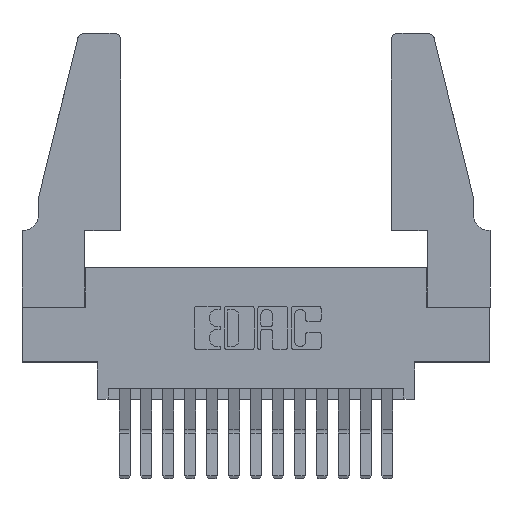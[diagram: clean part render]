
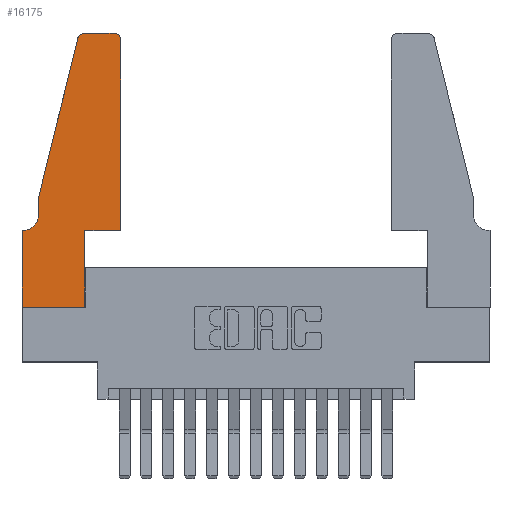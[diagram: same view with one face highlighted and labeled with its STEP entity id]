
A CAD part, top view. The second image highlights one B-rep face of the part: STEP entity #16175.
In plain terms, the highlighted planar face has unit normal (0, 0, 1).
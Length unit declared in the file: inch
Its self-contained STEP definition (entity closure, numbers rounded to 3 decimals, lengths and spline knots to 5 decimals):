
#160 = LINE ( 'NONE', #10211, #7240 ) ;
#206 = VERTEX_POINT ( 'NONE', #323 ) ;
#312 = CARTESIAN_POINT ( 'NONE',  ( 0.4205, 1.25, 0.37 ) ) ;
#323 = CARTESIAN_POINT ( 'NONE',  ( 0.2865, 0., 0.37 ) ) ;
#703 = EDGE_CURVE ( 'NONE', #14632, #4923, #6766, .T. ) ;
#1044 = EDGE_CURVE ( 'NONE', #5575, #206, #8657, .T. ) ;
#1192 = DIRECTION ( 'NONE',  ( 0., -1., 0. ) ) ;
#2066 = DIRECTION ( 'NONE',  ( -1., 0., 0. ) ) ;
#2116 = CARTESIAN_POINT ( 'NONE',  ( 0., 0., 0.37 ) ) ;
#2457 = VERTEX_POINT ( 'NONE', #15928 ) ;
#2574 = PLANE ( 'NONE',  #6379 ) ;
#2607 = ORIENTED_EDGE ( 'NONE', *, *, #14263, .T. ) ;
#2637 = CARTESIAN_POINT ( 'NONE',  ( 0.4505, 0.35, 0.37 ) ) ;
#2663 = VECTOR ( 'NONE', #8257, 39.37008 ) ;
#2886 = EDGE_CURVE ( 'NONE', #10358, #5575, #12281, .T. ) ;
#3018 = CARTESIAN_POINT ( 'NONE',  ( 0.0755, 0.5, 0.37 ) ) ;
#3720 = FACE_OUTER_BOUND ( 'NONE', #13090, .T. ) ;
#3921 = DIRECTION ( 'NONE',  ( 1., 0., 0. ) ) ;
#3925 = CARTESIAN_POINT ( 'NONE',  ( 0., 0.35, 0.37 ) ) ;
#4291 = ORIENTED_EDGE ( 'NONE', *, *, #4807, .T. ) ;
#4507 = DIRECTION ( 'NONE',  ( 0., 0., 1. ) ) ;
#4522 = CARTESIAN_POINT ( 'NONE',  ( 0., 0., 0.37 ) ) ;
#4807 = EDGE_CURVE ( 'NONE', #10381, #10608, #14722, .T. ) ;
#4842 = VECTOR ( 'NONE', #6902, 39.37008 ) ;
#4923 = VERTEX_POINT ( 'NONE', #10770 ) ;
#4931 = ORIENTED_EDGE ( 'NONE', *, *, #703, .T. ) ;
#5129 = CARTESIAN_POINT ( 'NONE',  ( 0.0755, 0.42, 0.37 ) ) ;
#5266 = CARTESIAN_POINT ( 'NONE',  ( 0.25487, 1.22718, 0.37 ) ) ;
#5298 = VERTEX_POINT ( 'NONE', #12648 ) ;
#5575 = VERTEX_POINT ( 'NONE', #14480 ) ;
#5789 = VECTOR ( 'NONE', #7447, 39.37008 ) ;
#6077 = CARTESIAN_POINT ( 'NONE',  ( 0.284, 1.22, 0.37 ) ) ;
#6230 = DIRECTION ( 'NONE',  ( 0., 0., -1. ) ) ;
#6379 = AXIS2_PLACEMENT_3D ( 'NONE', #6495, #11458, #3921 ) ;
#6452 = DIRECTION ( 'NONE',  ( 0., 1., 0. ) ) ;
#6495 = CARTESIAN_POINT ( 'NONE',  ( 0., 0.35, 0.37 ) ) ;
#6766 = LINE ( 'NONE', #14301, #9239 ) ;
#6902 = DIRECTION ( 'NONE',  ( 0., 1., 0. ) ) ;
#7240 = VECTOR ( 'NONE', #1192, 39.37008 ) ;
#7325 = DIRECTION ( 'NONE',  ( 1., 0., 0. ) ) ;
#7447 = DIRECTION ( 'NONE',  ( 1., 0., 0. ) ) ;
#7707 = ORIENTED_EDGE ( 'NONE', *, *, #11265, .T. ) ;
#8247 = ORIENTED_EDGE ( 'NONE', *, *, #15392, .T. ) ;
#8257 = DIRECTION ( 'NONE',  ( 1., 0., 0. ) ) ;
#8309 = CIRCLE ( 'NONE', #14732, 0.03 ) ;
#8619 = ORIENTED_EDGE ( 'NONE', *, *, #10227, .T. ) ;
#8657 = LINE ( 'NONE', #2116, #5789 ) ;
#8687 = CARTESIAN_POINT ( 'NONE',  ( 0.0755, 0.5, 0.37 ) ) ;
#8838 = LINE ( 'NONE', #15063, #14643 ) ;
#9239 = VECTOR ( 'NONE', #13051, 39.37008 ) ;
#9445 = LINE ( 'NONE', #15656, #2663 ) ;
#9787 = ORIENTED_EDGE ( 'NONE', *, *, #2886, .T. ) ;
#9834 = AXIS2_PLACEMENT_3D ( 'NONE', #13614, #6230, #14847 ) ;
#10174 = ORIENTED_EDGE ( 'NONE', *, *, #10321, .T. ) ;
#10211 = CARTESIAN_POINT ( 'NONE',  ( 0.0755, 0.5, 0.37 ) ) ;
#10227 = EDGE_CURVE ( 'NONE', #14513, #14608, #12912, .T. ) ;
#10321 = EDGE_CURVE ( 'NONE', #206, #2457, #8838, .T. ) ;
#10358 = VERTEX_POINT ( 'NONE', #3925 ) ;
#10381 = VERTEX_POINT ( 'NONE', #2637 ) ;
#10549 = CARTESIAN_POINT ( 'NONE',  ( 0.4505, 0.35, 0.37 ) ) ;
#10608 = VERTEX_POINT ( 'NONE', #13182 ) ;
#10770 = CARTESIAN_POINT ( 'NONE',  ( 0.284, 1.25, 0.37 ) ) ;
#10771 = AXIS2_PLACEMENT_3D ( 'NONE', #11965, #4507, #13225 ) ;
#11265 = EDGE_CURVE ( 'NONE', #10608, #14632, #14232, .T. ) ;
#11451 = VECTOR ( 'NONE', #2066, 39.37008 ) ;
#11458 = DIRECTION ( 'NONE',  ( 0., 0., 1. ) ) ;
#11562 = VERTEX_POINT ( 'NONE', #5129 ) ;
#11922 = ORIENTED_EDGE ( 'NONE', *, *, #13259, .T. ) ;
#11965 = CARTESIAN_POINT ( 'NONE',  ( 0.4205, 1.22, 0.37 ) ) ;
#12078 = EDGE_CURVE ( 'NONE', #11562, #5298, #14586, .T. ) ;
#12281 = LINE ( 'NONE', #4522, #15569 ) ;
#12428 = DIRECTION ( 'NONE',  ( -0.239, -0.971, 0. ) ) ;
#12527 = VECTOR ( 'NONE', #12428, 39.37008 ) ;
#12648 = CARTESIAN_POINT ( 'NONE',  ( 0.0055, 0.35, 0.37 ) ) ;
#12912 = LINE ( 'NONE', #8687, #12527 ) ;
#13051 = DIRECTION ( 'NONE',  ( -1., 0., 0. ) ) ;
#13081 = ORIENTED_EDGE ( 'NONE', *, *, #1044, .T. ) ;
#13090 = EDGE_LOOP ( 'NONE', ( #4931, #8247, #8619, #11922, #15594, #2607, #9787, #13081, #10174, #13471, #4291, #7707 ) ) ;
#13182 = CARTESIAN_POINT ( 'NONE',  ( 0.4505, 1.22, 0.37 ) ) ;
#13225 = DIRECTION ( 'NONE',  ( 1., 0., 0. ) ) ;
#13259 = EDGE_CURVE ( 'NONE', #14608, #11562, #160, .T. ) ;
#13471 = ORIENTED_EDGE ( 'NONE', *, *, #16425, .T. ) ;
#13614 = CARTESIAN_POINT ( 'NONE',  ( 0.0055, 0.42, 0.37 ) ) ;
#14232 = CIRCLE ( 'NONE', #10771, 0.03 ) ;
#14263 = EDGE_CURVE ( 'NONE', #5298, #10358, #15109, .T. ) ;
#14301 = CARTESIAN_POINT ( 'NONE',  ( 0.2605, 1.25, 0.37 ) ) ;
#14480 = CARTESIAN_POINT ( 'NONE',  ( 0., 0., 0.37 ) ) ;
#14513 = VERTEX_POINT ( 'NONE', #5266 ) ;
#14586 = CIRCLE ( 'NONE', #9834, 0.07 ) ;
#14608 = VERTEX_POINT ( 'NONE', #3018 ) ;
#14632 = VERTEX_POINT ( 'NONE', #312 ) ;
#14643 = VECTOR ( 'NONE', #6452, 39.37008 ) ;
#14703 = DIRECTION ( 'NONE',  ( 0., 0., 1. ) ) ;
#14722 = LINE ( 'NONE', #10549, #4842 ) ;
#14732 = AXIS2_PLACEMENT_3D ( 'NONE', #6077, #14703, #7325 ) ;
#14847 = DIRECTION ( 'NONE',  ( -1., 0., 0. ) ) ;
#15063 = CARTESIAN_POINT ( 'NONE',  ( 0.2865, 0.35, 0.37 ) ) ;
#15109 = LINE ( 'NONE', #15917, #11451 ) ;
#15392 = EDGE_CURVE ( 'NONE', #4923, #14513, #8309, .T. ) ;
#15569 = VECTOR ( 'NONE', #15830, 39.37008 ) ;
#15594 = ORIENTED_EDGE ( 'NONE', *, *, #12078, .T. ) ;
#15656 = CARTESIAN_POINT ( 'NONE',  ( 0.4505, 0.35, 0.37 ) ) ;
#15830 = DIRECTION ( 'NONE',  ( 0., -1., 0. ) ) ;
#15917 = CARTESIAN_POINT ( 'NONE',  ( 0.0755, 0.35, 0.37 ) ) ;
#15928 = CARTESIAN_POINT ( 'NONE',  ( 0.2865, 0.35, 0.37 ) ) ;
#16175 = ADVANCED_FACE ( 'NONE', ( #3720 ), #2574, .T. ) ;
#16425 = EDGE_CURVE ( 'NONE', #2457, #10381, #9445, .T. ) ;
